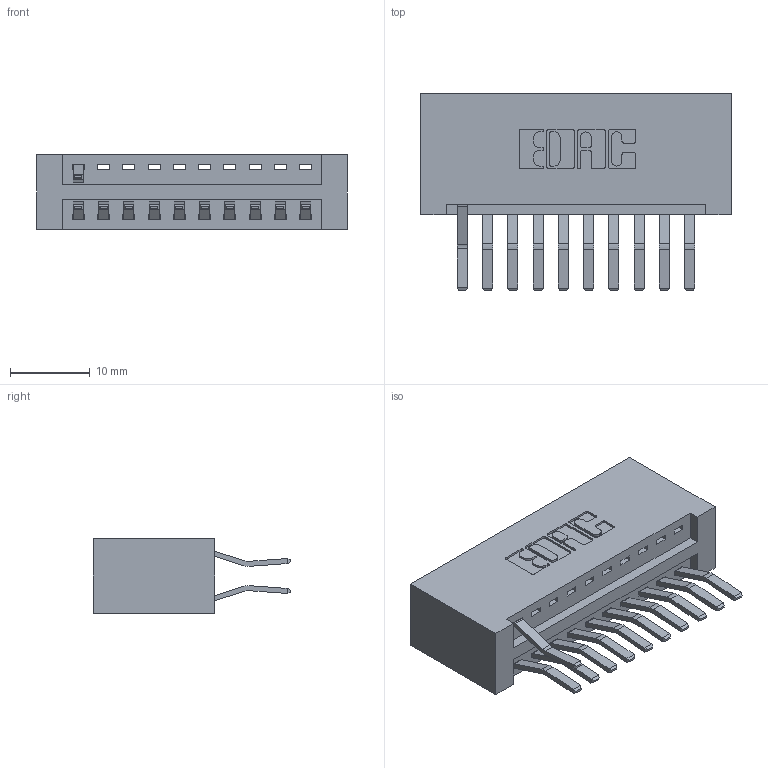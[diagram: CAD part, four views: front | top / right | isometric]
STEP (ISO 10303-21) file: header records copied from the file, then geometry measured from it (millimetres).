
FILE_DESCRIPTION (( 'STEP AP203' ), '1' );
FILE_NAME ('346-020-560-201.STEP', '2018-08-20T22:28:11', ( '' ), ( '' ), 'SwSTEP 2.0', 'SolidWorks 2016', '' );
FILE_SCHEMA (( 'CONFIG_CONTROL_DESIGN' ));
Length unit declared in the file: inch
Products named in the file (3): 346 Part_No Mounting Lugs; 345-292-001_560 Tail; 346-020-560-201
Assembly tree (12 placements, depth 2):
  346-020-560-201
    346 Part_No Mounting Lugs
    345-292-001_560 Tail  x11
Bounding box: 38.99 x 24.78 x 9.4 mm (x, y, z)
Volume: 4117.8 mm3; surface area: 5045.7 mm2
Topology: 12 solids, 12 shells, 762 faces, 2265 edges, 1494 vertices
Faces by surface type: plane 502, cylinder 260
Entity records: 10357 total; most frequent: CARTESIAN_POINT 1787, ORIENTED_EDGE 1730, DIRECTION 1615, EDGE_CURVE 865, VECTOR 697, LINE 697, VERTEX_POINT 574, AXIS2_PLACEMENT_3D 459
